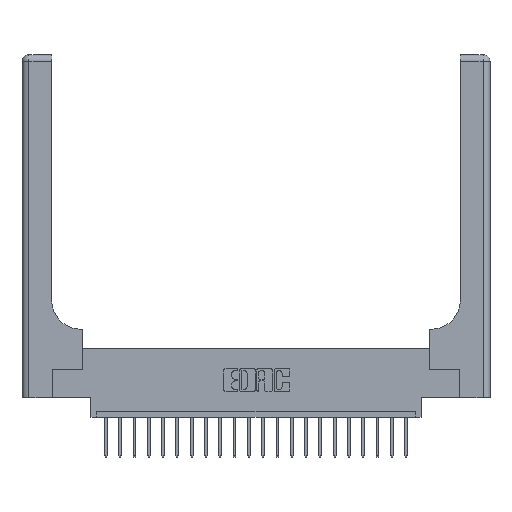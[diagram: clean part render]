
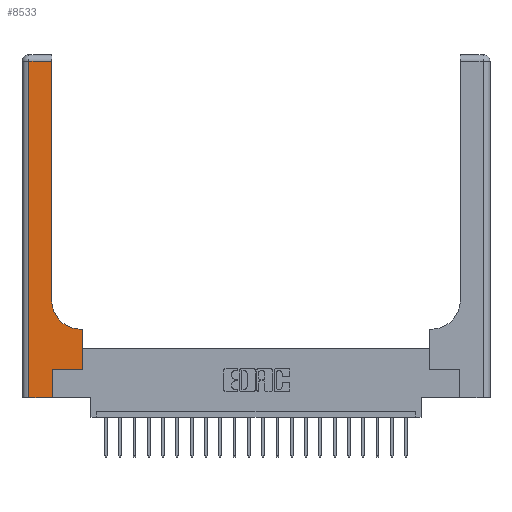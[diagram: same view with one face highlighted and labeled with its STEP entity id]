
A CAD part, top view. The second image highlights one B-rep face of the part: STEP entity #8533.
In plain terms, the highlighted planar face has unit normal (0, 0, 1).
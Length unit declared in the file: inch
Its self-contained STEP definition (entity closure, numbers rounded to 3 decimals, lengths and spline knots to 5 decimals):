
#90 = CARTESIAN_POINT ( 'NONE',  ( 0., 3., 0.37 ) ) ;
#391 = CARTESIAN_POINT ( 'NONE',  ( 0.26, 0.85, 0.37 ) ) ;
#596 = DIRECTION ( 'NONE',  ( -1., 0., 0. ) ) ;
#1099 = DIRECTION ( 'NONE',  ( 0., 1., 0. ) ) ;
#1190 = DIRECTION ( 'NONE',  ( 1., 0., 0. ) ) ;
#1503 = EDGE_CURVE ( 'NONE', #7644, #7771, #13357, .T. ) ;
#1773 = DIRECTION ( 'NONE',  ( -1., 0., 0. ) ) ;
#2031 = VERTEX_POINT ( 'NONE', #18662 ) ;
#2757 = CARTESIAN_POINT ( 'NONE',  ( 0.528, 0.6, 0.37 ) ) ;
#2849 = ORIENTED_EDGE ( 'NONE', *, *, #21587, .T. ) ;
#2987 = EDGE_CURVE ( 'NONE', #13905, #7270, #3629, .T. ) ;
#3499 = CARTESIAN_POINT ( 'NONE',  ( 0.265, 0., 0.37 ) ) ;
#3629 = LINE ( 'NONE', #20418, #15450 ) ;
#4082 = VERTEX_POINT ( 'NONE', #5191 ) ;
#4185 = EDGE_CURVE ( 'NONE', #7270, #4082, #10662, .T. ) ;
#4588 = VERTEX_POINT ( 'NONE', #10087 ) ;
#5013 = DIRECTION ( 'NONE',  ( 0., -1., 0. ) ) ;
#5191 = CARTESIAN_POINT ( 'NONE',  ( 0.51, 0.6, 0.37 ) ) ;
#5497 = DIRECTION ( 'NONE',  ( 0., 0., -1. ) ) ;
#5628 = VECTOR ( 'NONE', #1190, 39.37008 ) ;
#5855 = EDGE_CURVE ( 'NONE', #4082, #14711, #19456, .T. ) ;
#5896 = CARTESIAN_POINT ( 'NONE',  ( 0.528, 0.25, 0.37 ) ) ;
#6605 = ORIENTED_EDGE ( 'NONE', *, *, #16633, .T. ) ;
#7154 = ORIENTED_EDGE ( 'NONE', *, *, #2987, .T. ) ;
#7270 = VERTEX_POINT ( 'NONE', #2757 ) ;
#7644 = VERTEX_POINT ( 'NONE', #3499 ) ;
#7741 = DIRECTION ( 'NONE',  ( 1., 0., 0. ) ) ;
#7771 = VERTEX_POINT ( 'NONE', #14439 ) ;
#8527 = VECTOR ( 'NONE', #19769, 39.37008 ) ;
#8533 = ADVANCED_FACE ( 'NONE', ( #13591 ), #15272, .F. ) ;
#8551 = VERTEX_POINT ( 'NONE', #18519 ) ;
#9074 = CARTESIAN_POINT ( 'NONE',  ( 0., 2.94, 0.37 ) ) ;
#9654 = ORIENTED_EDGE ( 'NONE', *, *, #4185, .T. ) ;
#10087 = CARTESIAN_POINT ( 'NONE',  ( 0.26, 2.94, 0.37 ) ) ;
#10445 = DIRECTION ( 'NONE',  ( 0., 1., 0. ) ) ;
#10638 = EDGE_CURVE ( 'NONE', #4588, #8551, #13883, .T. ) ;
#10662 = LINE ( 'NONE', #15707, #18335 ) ;
#10688 = VECTOR ( 'NONE', #1099, 39.37008 ) ;
#11148 = LINE ( 'NONE', #19662, #8527 ) ;
#11722 = CARTESIAN_POINT ( 'NONE',  ( 0.06, 3., 0.37 ) ) ;
#12318 = DIRECTION ( 'NONE',  ( 1., 0., 0. ) ) ;
#12454 = DIRECTION ( 'NONE',  ( -1., 0., 0. ) ) ;
#13255 = CARTESIAN_POINT ( 'NONE',  ( 0.265, 0., 0.37 ) ) ;
#13357 = LINE ( 'NONE', #13255, #10688 ) ;
#13591 = FACE_OUTER_BOUND ( 'NONE', #21226, .T. ) ;
#13883 = LINE ( 'NONE', #9074, #16702 ) ;
#13905 = VERTEX_POINT ( 'NONE', #5896 ) ;
#14099 = ORIENTED_EDGE ( 'NONE', *, *, #19708, .T. ) ;
#14439 = CARTESIAN_POINT ( 'NONE',  ( 0.265, 0.25, 0.37 ) ) ;
#14693 = CARTESIAN_POINT ( 'NONE',  ( 0., 0., 0.37 ) ) ;
#14711 = VERTEX_POINT ( 'NONE', #391 ) ;
#14800 = LINE ( 'NONE', #14693, #5628 ) ;
#15272 = PLANE ( 'NONE',  #15937 ) ;
#15365 = VECTOR ( 'NONE', #5013, 39.37008 ) ;
#15450 = VECTOR ( 'NONE', #10445, 39.37008 ) ;
#15656 = VECTOR ( 'NONE', #7741, 39.37008 ) ;
#15707 = CARTESIAN_POINT ( 'NONE',  ( 0.26, 0.6, 0.37 ) ) ;
#15937 = AXIS2_PLACEMENT_3D ( 'NONE', #90, #20330, #1773 ) ;
#16359 = CARTESIAN_POINT ( 'NONE',  ( 0.265, 0.25, 0.37 ) ) ;
#16621 = AXIS2_PLACEMENT_3D ( 'NONE', #20838, #5497, #12318 ) ;
#16633 = EDGE_CURVE ( 'NONE', #2031, #7644, #14800, .T. ) ;
#16702 = VECTOR ( 'NONE', #596, 39.37008 ) ;
#17921 = ORIENTED_EDGE ( 'NONE', *, *, #1503, .T. ) ;
#17958 = EDGE_CURVE ( 'NONE', #14711, #4588, #11148, .T. ) ;
#18335 = VECTOR ( 'NONE', #12454, 39.37008 ) ;
#18519 = CARTESIAN_POINT ( 'NONE',  ( 0.06, 2.94, 0.37 ) ) ;
#18662 = CARTESIAN_POINT ( 'NONE',  ( 0.06, 0., 0.37 ) ) ;
#19181 = ORIENTED_EDGE ( 'NONE', *, *, #17958, .T. ) ;
#19377 = ORIENTED_EDGE ( 'NONE', *, *, #10638, .T. ) ;
#19456 = CIRCLE ( 'NONE', #16621, 0.25 ) ;
#19662 = CARTESIAN_POINT ( 'NONE',  ( 0.26, 3., 0.37 ) ) ;
#19708 = EDGE_CURVE ( 'NONE', #7771, #13905, #21633, .T. ) ;
#19769 = DIRECTION ( 'NONE',  ( 0., 1., 0. ) ) ;
#20330 = DIRECTION ( 'NONE',  ( 0., 0., -1. ) ) ;
#20345 = LINE ( 'NONE', #11722, #15365 ) ;
#20418 = CARTESIAN_POINT ( 'NONE',  ( 0.528, 0.25, 0.37 ) ) ;
#20838 = CARTESIAN_POINT ( 'NONE',  ( 0.51, 0.85, 0.37 ) ) ;
#21226 = EDGE_LOOP ( 'NONE', ( #19181, #19377, #2849, #6605, #17921, #14099, #7154, #9654, #21919 ) ) ;
#21587 = EDGE_CURVE ( 'NONE', #8551, #2031, #20345, .T. ) ;
#21633 = LINE ( 'NONE', #16359, #15656 ) ;
#21919 = ORIENTED_EDGE ( 'NONE', *, *, #5855, .T. ) ;
